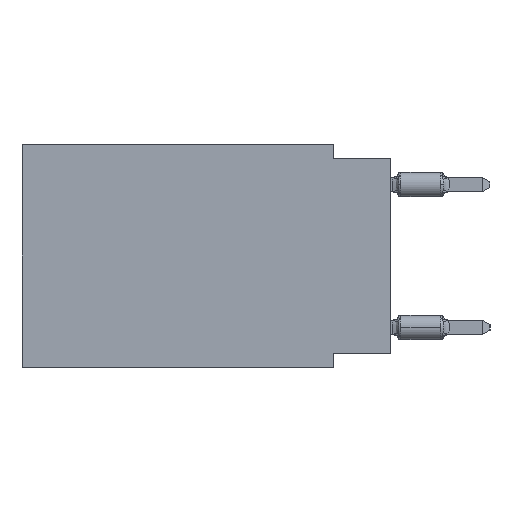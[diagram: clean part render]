
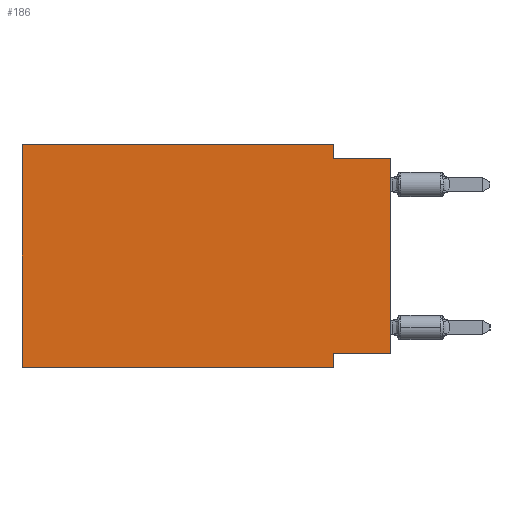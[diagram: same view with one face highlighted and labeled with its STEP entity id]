
A CAD part, left-side view. The second image highlights one B-rep face of the part: STEP entity #186.
In plain terms, the highlighted planar face has unit normal (-1, 0, 0).
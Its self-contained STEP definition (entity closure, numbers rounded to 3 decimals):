
#186 = ADVANCED_FACE ( 'NONE', ( #9234 ), #32816, .F. ) ;
#482 = AXIS2_PLACEMENT_3D ( 'NONE', #946, #33207, #18518 ) ;
#743 = VECTOR ( 'NONE', #30907, 1000. ) ;
#946 = CARTESIAN_POINT ( 'NONE',  ( 0., 16.383, 0. ) ) ;
#1660 = DIRECTION ( 'NONE',  ( 0., -1., 0. ) ) ;
#2136 = VERTEX_POINT ( 'NONE', #36287 ) ;
#2589 = EDGE_LOOP ( 'NONE', ( #8927, #25146, #34034, #10800, #27041, #5604, #14614, #35779 ) ) ;
#3151 = CARTESIAN_POINT ( 'NONE',  ( 0., 2.54, 0. ) ) ;
#5604 = ORIENTED_EDGE ( 'NONE', *, *, #7217, .T. ) ;
#6804 = DIRECTION ( 'NONE',  ( 0., 1., 0. ) ) ;
#7217 = EDGE_CURVE ( 'NONE', #37635, #2136, #25637, .T. ) ;
#7328 = LINE ( 'NONE', #22415, #743 ) ;
#8266 = VECTOR ( 'NONE', #30795, 1000. ) ;
#8274 = CARTESIAN_POINT ( 'NONE',  ( 0., 2.54, -9.271 ) ) ;
#8313 = DIRECTION ( 'NONE',  ( 0., 0., -1. ) ) ;
#8613 = CARTESIAN_POINT ( 'NONE',  ( 0., 0., -9.271 ) ) ;
#8927 = ORIENTED_EDGE ( 'NONE', *, *, #34837, .T. ) ;
#9234 = FACE_OUTER_BOUND ( 'NONE', #2589, .T. ) ;
#9477 = VERTEX_POINT ( 'NONE', #19987 ) ;
#10704 = VERTEX_POINT ( 'NONE', #8274 ) ;
#10800 = ORIENTED_EDGE ( 'NONE', *, *, #30559, .F. ) ;
#11013 = CARTESIAN_POINT ( 'NONE',  ( 0., 2.54, 0. ) ) ;
#11274 = CARTESIAN_POINT ( 'NONE',  ( 0., 0., 0. ) ) ;
#12560 = VECTOR ( 'NONE', #8313, 1000. ) ;
#14614 = ORIENTED_EDGE ( 'NONE', *, *, #37406, .F. ) ;
#14620 = CARTESIAN_POINT ( 'NONE',  ( 0., 0., -0.635 ) ) ;
#15228 = EDGE_CURVE ( 'NONE', #37635, #9477, #7328, .T. ) ;
#16811 = LINE ( 'NONE', #11013, #12560 ) ;
#18518 = DIRECTION ( 'NONE',  ( 0., 0., -1. ) ) ;
#19346 = DIRECTION ( 'NONE',  ( 0., 0., -1. ) ) ;
#19987 = CARTESIAN_POINT ( 'NONE',  ( 0., 16.383, 0. ) ) ;
#20152 = VECTOR ( 'NONE', #22724, 1000. ) ;
#20487 = VECTOR ( 'NONE', #6804, 1000. ) ;
#20595 = VECTOR ( 'NONE', #34523, 1000. ) ;
#21232 = EDGE_CURVE ( 'NONE', #22089, #23628, #16811, .T. ) ;
#21665 = EDGE_CURVE ( 'NONE', #23628, #25852, #38026, .T. ) ;
#21879 = LINE ( 'NONE', #27100, #20487 ) ;
#22089 = VERTEX_POINT ( 'NONE', #3151 ) ;
#22250 = CARTESIAN_POINT ( 'NONE',  ( 0., 2.54, -9.906 ) ) ;
#22415 = CARTESIAN_POINT ( 'NONE',  ( 0., 16.383, 0. ) ) ;
#22724 = DIRECTION ( 'NONE',  ( 0., 0., 1. ) ) ;
#22879 = VECTOR ( 'NONE', #19346, 1000. ) ;
#23628 = VERTEX_POINT ( 'NONE', #36880 ) ;
#25146 = ORIENTED_EDGE ( 'NONE', *, *, #21665, .F. ) ;
#25404 = LINE ( 'NONE', #34487, #26972 ) ;
#25637 = LINE ( 'NONE', #26008, #20595 ) ;
#25852 = VERTEX_POINT ( 'NONE', #26702 ) ;
#26008 = CARTESIAN_POINT ( 'NONE',  ( 0., 16.383, -9.906 ) ) ;
#26038 = EDGE_CURVE ( 'NONE', #30257, #10704, #21879, .T. ) ;
#26464 = CARTESIAN_POINT ( 'NONE',  ( 0., 16.383, -9.906 ) ) ;
#26702 = CARTESIAN_POINT ( 'NONE',  ( 0., 0., -0.635 ) ) ;
#26972 = VECTOR ( 'NONE', #1660, 1000. ) ;
#27041 = ORIENTED_EDGE ( 'NONE', *, *, #15228, .F. ) ;
#27100 = CARTESIAN_POINT ( 'NONE',  ( 0., 0., -9.271 ) ) ;
#30257 = VERTEX_POINT ( 'NONE', #8613 ) ;
#30559 = EDGE_CURVE ( 'NONE', #9477, #22089, #25404, .T. ) ;
#30795 = DIRECTION ( 'NONE',  ( 0., -1., 0. ) ) ;
#30907 = DIRECTION ( 'NONE',  ( 0., 0., 1. ) ) ;
#32816 = PLANE ( 'NONE',  #482 ) ;
#33207 = DIRECTION ( 'NONE',  ( 1., 0., 0. ) ) ;
#34034 = ORIENTED_EDGE ( 'NONE', *, *, #21232, .F. ) ;
#34487 = CARTESIAN_POINT ( 'NONE',  ( 0., 16.383, 0. ) ) ;
#34523 = DIRECTION ( 'NONE',  ( 0., -1., 0. ) ) ;
#34837 = EDGE_CURVE ( 'NONE', #30257, #25852, #37772, .T. ) ;
#35779 = ORIENTED_EDGE ( 'NONE', *, *, #26038, .F. ) ;
#36287 = CARTESIAN_POINT ( 'NONE',  ( 0., 2.54, -9.906 ) ) ;
#36880 = CARTESIAN_POINT ( 'NONE',  ( 0., 2.54, -0.635 ) ) ;
#36929 = LINE ( 'NONE', #22250, #22879 ) ;
#37406 = EDGE_CURVE ( 'NONE', #10704, #2136, #36929, .T. ) ;
#37635 = VERTEX_POINT ( 'NONE', #26464 ) ;
#37772 = LINE ( 'NONE', #11274, #20152 ) ;
#38026 = LINE ( 'NONE', #14620, #8266 ) ;
